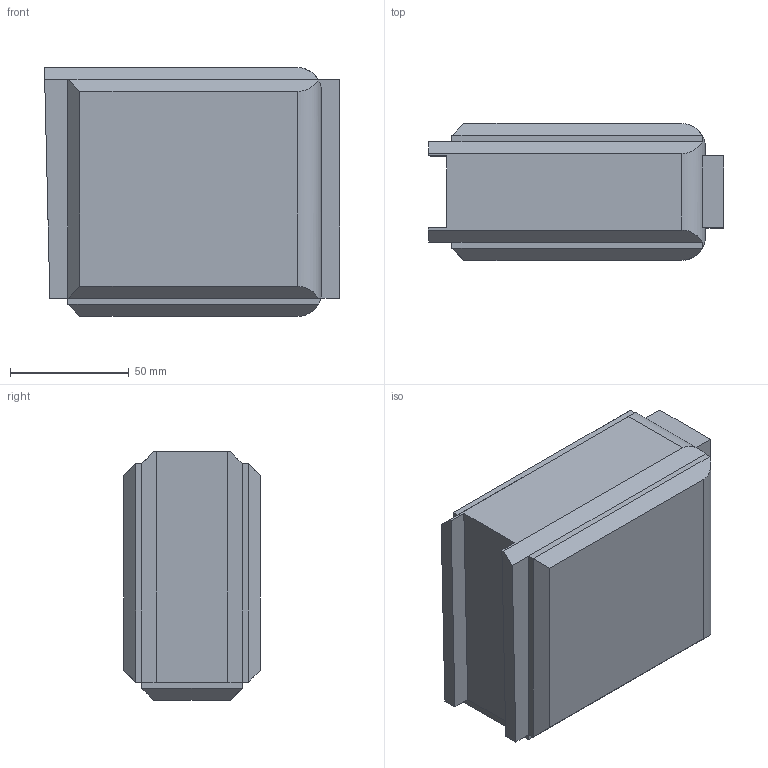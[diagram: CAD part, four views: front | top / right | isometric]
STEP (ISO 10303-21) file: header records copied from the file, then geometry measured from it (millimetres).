
FILE_DESCRIPTION (( 'STEP AP214' ), '1' );
FILE_NAME ('hydrastocky2.STEP', '2013-07-04T02:36:11', ( '' ), ( '' ), 'SwSTEP 2.0', 'SolidWorks 2012', '' );
FILE_SCHEMA (( 'AUTOMOTIVE_DESIGN' ));
Length unit declared in the file: inch
Products named in the file (1): hydrastocky2
Bounding box: 124.16 x 57.48 x 104.59 mm (x, y, z)
Volume: 636566 mm3; surface area: 47002.8 mm2
Topology: 1 solids, 1 shells, 44 faces, 106 edges, 64 vertices
Faces by surface type: plane 40, cylinder 4
Entity records: 1278 total; most frequent: CARTESIAN_POINT 251, ORIENTED_EDGE 212, DIRECTION 192, EDGE_CURVE 106, VECTOR 86, LINE 86, VERTEX_POINT 64, AXIS2_PLACEMENT_3D 53
